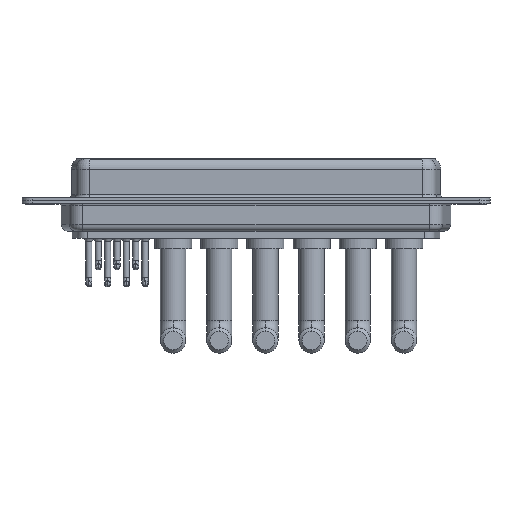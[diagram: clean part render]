
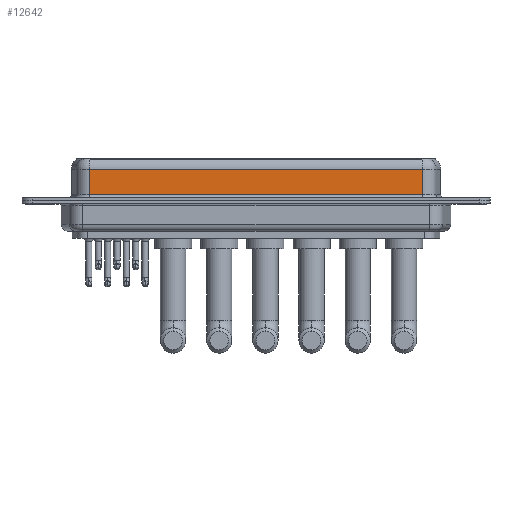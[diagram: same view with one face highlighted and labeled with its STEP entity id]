
A CAD part, front view. The second image highlights one B-rep face of the part: STEP entity #12642.
In plain terms, the highlighted planar face has unit normal (0, -1, 0).
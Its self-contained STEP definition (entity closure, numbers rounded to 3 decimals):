
#24 = FACE_OUTER_BOUND ( 'NONE', #5342, .T. ) ;
#136 = VECTOR ( 'NONE', #2965, 1000. ) ;
#1448 = LINE ( 'NONE', #15924, #12779 ) ;
#2661 = CARTESIAN_POINT ( 'NONE',  ( 56.462, -3.95, 0.9 ) ) ;
#2965 = DIRECTION ( 'NONE',  ( 0., 0., -1. ) ) ;
#3536 = ORIENTED_EDGE ( 'NONE', *, *, #3862, .T. ) ;
#3599 = DIRECTION ( 'NONE',  ( 1., 0., 0. ) ) ;
#3862 = EDGE_CURVE ( 'NONE', #12609, #7963, #10153, .T. ) ;
#4060 = DIRECTION ( 'NONE',  ( 0., 0., 1. ) ) ;
#4080 = VECTOR ( 'NONE', #5276, 1000. ) ;
#4086 = VERTEX_POINT ( 'NONE', #7427 ) ;
#4138 = LINE ( 'NONE', #9275, #136 ) ;
#5276 = DIRECTION ( 'NONE',  ( -1., 0., 0. ) ) ;
#5342 = EDGE_LOOP ( 'NONE', ( #8902, #13612, #5417, #3536 ) ) ;
#5411 = VECTOR ( 'NONE', #3599, 1000. ) ;
#5417 = ORIENTED_EDGE ( 'NONE', *, *, #16460, .T. ) ;
#7427 = CARTESIAN_POINT ( 'NONE',  ( 56.462, -3.95, 4.65 ) ) ;
#7963 = VERTEX_POINT ( 'NONE', #8277 ) ;
#8006 = DIRECTION ( 'NONE',  ( 0., 1., 0. ) ) ;
#8277 = CARTESIAN_POINT ( 'NONE',  ( 56.462, -3.95, 0.9 ) ) ;
#8378 = EDGE_CURVE ( 'NONE', #4086, #7963, #1448, .T. ) ;
#8816 = CARTESIAN_POINT ( 'NONE',  ( 56.462, -3.95, 4.65 ) ) ;
#8902 = ORIENTED_EDGE ( 'NONE', *, *, #8378, .F. ) ;
#9201 = AXIS2_PLACEMENT_3D ( 'NONE', #11873, #8006, #4060 ) ;
#9275 = CARTESIAN_POINT ( 'NONE',  ( 7.038, -3.95, 6.4 ) ) ;
#10153 = LINE ( 'NONE', #2661, #5411 ) ;
#10547 = PLANE ( 'NONE',  #9201 ) ;
#10717 = DIRECTION ( 'NONE',  ( 0., 0., -1. ) ) ;
#11348 = LINE ( 'NONE', #8816, #4080 ) ;
#11873 = CARTESIAN_POINT ( 'NONE',  ( 56.462, -3.95, 6.4 ) ) ;
#11957 = CARTESIAN_POINT ( 'NONE',  ( 7.038, -3.95, 4.65 ) ) ;
#12153 = EDGE_CURVE ( 'NONE', #4086, #16446, #11348, .T. ) ;
#12609 = VERTEX_POINT ( 'NONE', #15506 ) ;
#12642 = ADVANCED_FACE ( 'NONE', ( #24 ), #10547, .F. ) ;
#12779 = VECTOR ( 'NONE', #10717, 1000. ) ;
#13612 = ORIENTED_EDGE ( 'NONE', *, *, #12153, .T. ) ;
#15506 = CARTESIAN_POINT ( 'NONE',  ( 7.038, -3.95, 0.9 ) ) ;
#15924 = CARTESIAN_POINT ( 'NONE',  ( 56.462, -3.95, 6.4 ) ) ;
#16446 = VERTEX_POINT ( 'NONE', #11957 ) ;
#16460 = EDGE_CURVE ( 'NONE', #16446, #12609, #4138, .T. ) ;
